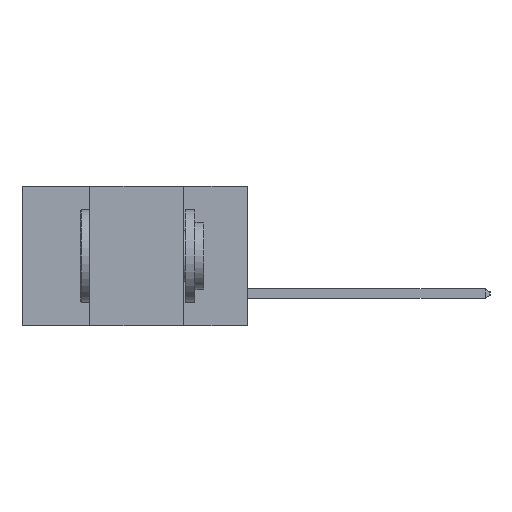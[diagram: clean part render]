
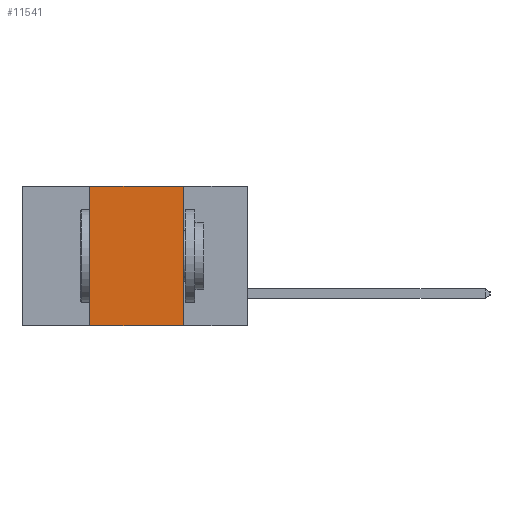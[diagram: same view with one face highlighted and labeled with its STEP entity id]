
A CAD part, left-side view. The second image highlights one B-rep face of the part: STEP entity #11541.
In plain terms, the highlighted planar face has unit normal (-1, 0, 0).
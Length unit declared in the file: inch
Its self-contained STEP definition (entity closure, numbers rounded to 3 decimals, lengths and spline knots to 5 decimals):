
#531 = DIRECTION ( 'NONE',  ( 0., -1., 0. ) ) ;
#1039 = CARTESIAN_POINT ( 'NONE',  ( 0., 0.6, 0. ) ) ;
#1077 = VERTEX_POINT ( 'NONE', #12786 ) ;
#1491 = VERTEX_POINT ( 'NONE', #4873 ) ;
#2726 = CARTESIAN_POINT ( 'NONE',  ( 0., 0.42, 0. ) ) ;
#3365 = LINE ( 'NONE', #4809, #15562 ) ;
#3561 = PLANE ( 'NONE',  #10998 ) ;
#4809 = CARTESIAN_POINT ( 'NONE',  ( 0., 0.17, -0.37 ) ) ;
#4832 = DIRECTION ( 'NONE',  ( 0., 0., -1. ) ) ;
#4873 = CARTESIAN_POINT ( 'NONE',  ( 0., 0.17, -0.37 ) ) ;
#5418 = EDGE_CURVE ( 'NONE', #7673, #10561, #11504, .T. ) ;
#5530 = CARTESIAN_POINT ( 'NONE',  ( 0., 0.6, -0.37 ) ) ;
#5613 = CARTESIAN_POINT ( 'NONE',  ( 0., 0.42, -0.37 ) ) ;
#5787 = CARTESIAN_POINT ( 'NONE',  ( 0., 0.6, 0. ) ) ;
#5965 = ORIENTED_EDGE ( 'NONE', *, *, #5418, .F. ) ;
#6349 = ORIENTED_EDGE ( 'NONE', *, *, #9530, .F. ) ;
#6582 = LINE ( 'NONE', #5530, #12683 ) ;
#7043 = DIRECTION ( 'NONE',  ( 0., -1., 0. ) ) ;
#7185 = DIRECTION ( 'NONE',  ( 0., 0., 1. ) ) ;
#7238 = CARTESIAN_POINT ( 'NONE',  ( 0., 0.42, -0.37 ) ) ;
#7673 = VERTEX_POINT ( 'NONE', #5613 ) ;
#7720 = FACE_OUTER_BOUND ( 'NONE', #11235, .T. ) ;
#8897 = VECTOR ( 'NONE', #7043, 39.37008 ) ;
#9279 = LINE ( 'NONE', #5787, #8897 ) ;
#9530 = EDGE_CURVE ( 'NONE', #10561, #1077, #9279, .T. ) ;
#9775 = ORIENTED_EDGE ( 'NONE', *, *, #15464, .T. ) ;
#10352 = EDGE_CURVE ( 'NONE', #1077, #1491, #3365, .T. ) ;
#10561 = VERTEX_POINT ( 'NONE', #2726 ) ;
#10998 = AXIS2_PLACEMENT_3D ( 'NONE', #1039, #12213, #4832 ) ;
#11235 = EDGE_LOOP ( 'NONE', ( #13197, #6349, #5965, #9775 ) ) ;
#11504 = LINE ( 'NONE', #7238, #14226 ) ;
#11541 = ADVANCED_FACE ( 'NONE', ( #7720 ), #3561, .F. ) ;
#12213 = DIRECTION ( 'NONE',  ( 1., 0., 0. ) ) ;
#12683 = VECTOR ( 'NONE', #531, 39.37008 ) ;
#12786 = CARTESIAN_POINT ( 'NONE',  ( 0., 0.17, 0. ) ) ;
#13197 = ORIENTED_EDGE ( 'NONE', *, *, #10352, .F. ) ;
#14226 = VECTOR ( 'NONE', #7185, 39.37008 ) ;
#14541 = DIRECTION ( 'NONE',  ( 0., 0., -1. ) ) ;
#15464 = EDGE_CURVE ( 'NONE', #7673, #1491, #6582, .T. ) ;
#15562 = VECTOR ( 'NONE', #14541, 39.37008 ) ;
